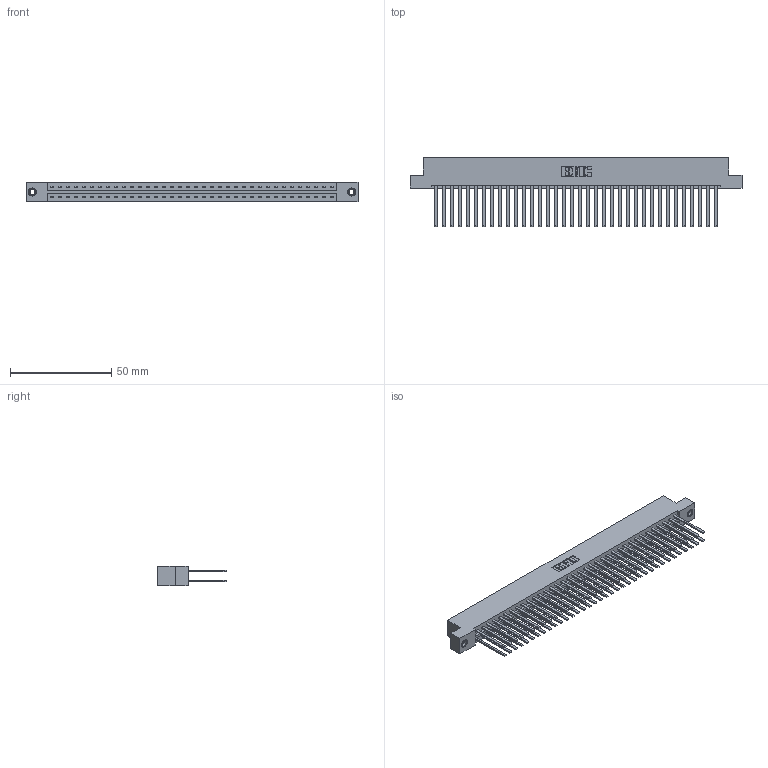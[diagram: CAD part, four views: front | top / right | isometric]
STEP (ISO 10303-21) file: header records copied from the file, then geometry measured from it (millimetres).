
FILE_DESCRIPTION (( 'STEP AP203' ), '1' );
FILE_NAME ('833-072-544-207.STEP', '2020-06-05T14:35:38', ( '' ), ( '' ), 'SwSTEP 2.0', 'SolidWorks 2020', '' );
FILE_SCHEMA (( 'CONFIG_CONTROL_DESIGN' ));
Length unit declared in the file: inch
Products named in the file (4): 345-250-001_345-250-005-103; 833-072-544-207; 833 Part_Flush - .156 Dia - TI; 345-292-001_345-293-144
Assembly tree (75 placements, depth 2):
  833-072-544-207
    833 Part_Flush - .156 Dia - TI
    345-292-001_345-293-144  x72
    345-250-001_345-250-005-103  x2
Bounding box: 164.19 x 34.3 x 9.4 mm (x, y, z)
Volume: 17702.1 mm3; surface area: 24147.6 mm2
Topology: 75 solids, 75 shells, 3486 faces, 10311 edges, 6770 vertices
Faces by surface type: plane 2406, cylinder 1064, cone 12, torus 4
Entity records: 24938 total; most frequent: CARTESIAN_POINT 4121, ORIENTED_EDGE 4050, DIRECTION 3559, EDGE_CURVE 2025, VECTOR 1881, LINE 1881, VERTEX_POINT 1344, AXIS2_PLACEMENT_3D 839
